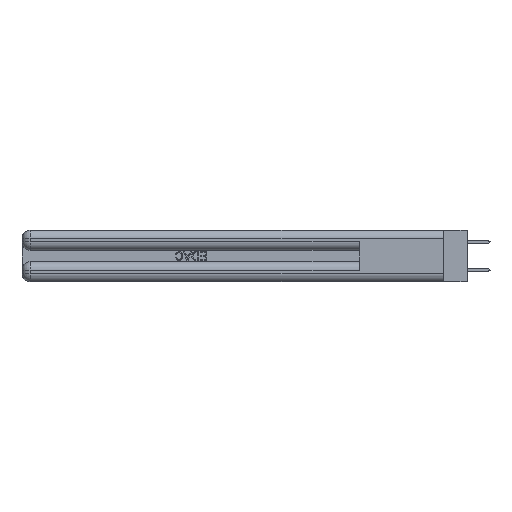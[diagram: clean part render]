
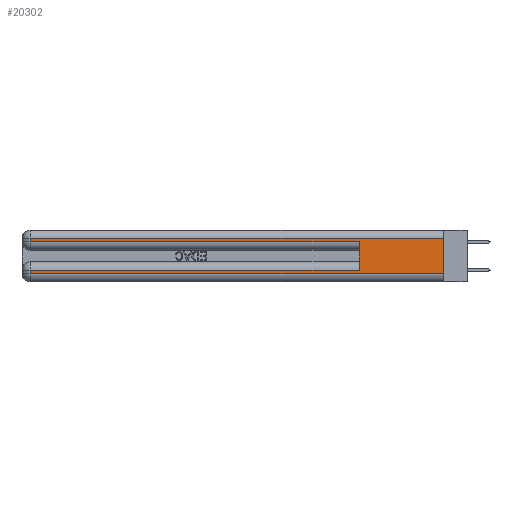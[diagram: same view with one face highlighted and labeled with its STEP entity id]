
A CAD part, left-side view. The second image highlights one B-rep face of the part: STEP entity #20302.
In plain terms, the highlighted planar face has unit normal (-1, 0, 0).
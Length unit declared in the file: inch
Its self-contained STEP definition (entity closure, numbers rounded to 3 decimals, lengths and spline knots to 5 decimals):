
#874 = ORIENTED_EDGE ( 'NONE', *, *, #13210, .T. ) ;
#1080 = CARTESIAN_POINT ( 'NONE',  ( 0., 0., 0.085 ) ) ;
#1847 = ORIENTED_EDGE ( 'NONE', *, *, #12623, .T. ) ;
#2276 = FACE_OUTER_BOUND ( 'NONE', #15755, .T. ) ;
#2787 = CARTESIAN_POINT ( 'NONE',  ( 0., 2.94, 0.37 ) ) ;
#3057 = AXIS2_PLACEMENT_3D ( 'NONE', #31570, #16886, #24153 ) ;
#3696 = VECTOR ( 'NONE', #37205, 39.37008 ) ;
#4658 = VERTEX_POINT ( 'NONE', #15935 ) ;
#4948 = LINE ( 'NONE', #10289, #35405 ) ;
#6013 = CARTESIAN_POINT ( 'NONE',  ( 0., 2.94, 0.06 ) ) ;
#6285 = LINE ( 'NONE', #2787, #8018 ) ;
#7440 = ORIENTED_EDGE ( 'NONE', *, *, #16015, .T. ) ;
#7564 = DIRECTION ( 'NONE',  ( 0., -1., 0. ) ) ;
#8018 = VECTOR ( 'NONE', #10205, 39.37008 ) ;
#8809 = ORIENTED_EDGE ( 'NONE', *, *, #9563, .T. ) ;
#9337 = CARTESIAN_POINT ( 'NONE',  ( 0., 0., 0.06 ) ) ;
#9563 = EDGE_CURVE ( 'NONE', #40974, #4658, #6285, .T. ) ;
#10205 = DIRECTION ( 'NONE',  ( 0., 0., -1. ) ) ;
#10289 = CARTESIAN_POINT ( 'NONE',  ( 0., 0., 0.06 ) ) ;
#11094 = LINE ( 'NONE', #36818, #38733 ) ;
#11102 = EDGE_CURVE ( 'NONE', #44650, #30387, #21465, .T. ) ;
#12623 = EDGE_CURVE ( 'NONE', #39084, #30387, #4948, .T. ) ;
#13068 = LINE ( 'NONE', #29678, #27781 ) ;
#13210 = EDGE_CURVE ( 'NONE', #44650, #40974, #39304, .T. ) ;
#13961 = CARTESIAN_POINT ( 'NONE',  ( 0., 2.94, 0.31 ) ) ;
#15755 = EDGE_LOOP ( 'NONE', ( #24081, #874, #8809, #40913, #24427, #42804, #7440, #1847 ) ) ;
#15935 = CARTESIAN_POINT ( 'NONE',  ( 0., 2.94, 0.285 ) ) ;
#16015 = EDGE_CURVE ( 'NONE', #18036, #39084, #41581, .T. ) ;
#16406 = PLANE ( 'NONE',  #3057 ) ;
#16886 = DIRECTION ( 'NONE',  ( 1., 0., 0. ) ) ;
#17402 = EDGE_CURVE ( 'NONE', #22903, #18036, #41546, .T. ) ;
#18036 = VERTEX_POINT ( 'NONE', #21234 ) ;
#18671 = DIRECTION ( 'NONE',  ( 0., 0., 1. ) ) ;
#19640 = CARTESIAN_POINT ( 'NONE',  ( 0., 0.6, 0.285 ) ) ;
#20302 = ADVANCED_FACE ( 'NONE', ( #2276 ), #16406, .F. ) ;
#20596 = CARTESIAN_POINT ( 'NONE',  ( 0., 2.94, 0.37 ) ) ;
#20853 = DIRECTION ( 'NONE',  ( 0., -1., 0. ) ) ;
#20878 = VECTOR ( 'NONE', #25924, 39.37008 ) ;
#21234 = CARTESIAN_POINT ( 'NONE',  ( 0., 2.94, 0.085 ) ) ;
#21239 = CARTESIAN_POINT ( 'NONE',  ( 0., 0., 0.37 ) ) ;
#21410 = CARTESIAN_POINT ( 'NONE',  ( 0., 0., 0.31 ) ) ;
#21465 = LINE ( 'NONE', #21239, #20878 ) ;
#22759 = CARTESIAN_POINT ( 'NONE',  ( 0., 0., 0.31 ) ) ;
#22903 = VERTEX_POINT ( 'NONE', #44570 ) ;
#24081 = ORIENTED_EDGE ( 'NONE', *, *, #11102, .F. ) ;
#24153 = DIRECTION ( 'NONE',  ( 0., 0., -1. ) ) ;
#24427 = ORIENTED_EDGE ( 'NONE', *, *, #43797, .F. ) ;
#25924 = DIRECTION ( 'NONE',  ( 0., 0., -1. ) ) ;
#27781 = VECTOR ( 'NONE', #7564, 39.37008 ) ;
#27820 = EDGE_CURVE ( 'NONE', #4658, #46504, #13068, .T. ) ;
#29678 = CARTESIAN_POINT ( 'NONE',  ( 0., 0., 0.285 ) ) ;
#30387 = VERTEX_POINT ( 'NONE', #9337 ) ;
#31570 = CARTESIAN_POINT ( 'NONE',  ( 0., 0., 0.37 ) ) ;
#32565 = VECTOR ( 'NONE', #45701, 39.37008 ) ;
#33855 = DIRECTION ( 'NONE',  ( 0., 1., 0. ) ) ;
#34231 = VECTOR ( 'NONE', #33855, 39.37008 ) ;
#35405 = VECTOR ( 'NONE', #20853, 39.37008 ) ;
#36818 = CARTESIAN_POINT ( 'NONE',  ( 0., 0.6, 0.145 ) ) ;
#37205 = DIRECTION ( 'NONE',  ( 0., 1., 0. ) ) ;
#38733 = VECTOR ( 'NONE', #18671, 39.37008 ) ;
#39084 = VERTEX_POINT ( 'NONE', #6013 ) ;
#39304 = LINE ( 'NONE', #21410, #34231 ) ;
#40913 = ORIENTED_EDGE ( 'NONE', *, *, #27820, .T. ) ;
#40974 = VERTEX_POINT ( 'NONE', #13961 ) ;
#41546 = LINE ( 'NONE', #1080, #3696 ) ;
#41581 = LINE ( 'NONE', #20596, #32565 ) ;
#42804 = ORIENTED_EDGE ( 'NONE', *, *, #17402, .T. ) ;
#43797 = EDGE_CURVE ( 'NONE', #22903, #46504, #11094, .T. ) ;
#44570 = CARTESIAN_POINT ( 'NONE',  ( 0., 0.6, 0.085 ) ) ;
#44650 = VERTEX_POINT ( 'NONE', #22759 ) ;
#45701 = DIRECTION ( 'NONE',  ( 0., 0., -1. ) ) ;
#46504 = VERTEX_POINT ( 'NONE', #19640 ) ;
